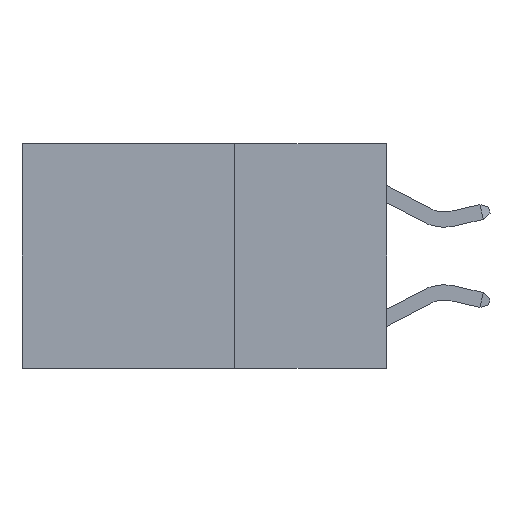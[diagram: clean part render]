
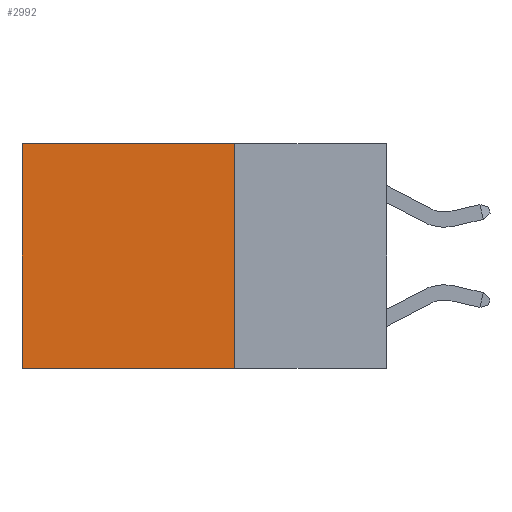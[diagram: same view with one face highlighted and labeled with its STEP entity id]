
A CAD part, left-side view. The second image highlights one B-rep face of the part: STEP entity #2992.
In plain terms, the highlighted planar face has unit normal (-1, 0, 0).
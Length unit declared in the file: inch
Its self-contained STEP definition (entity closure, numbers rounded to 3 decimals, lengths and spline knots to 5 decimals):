
#8 = VECTOR ( 'NONE', #3500, 39.37008 ) ;
#71 = VERTEX_POINT ( 'NONE', #1092 ) ;
#175 = ORIENTED_EDGE ( 'NONE', *, *, #10631, .F. ) ;
#311 = VECTOR ( 'NONE', #3768, 39.37008 ) ;
#1005 = LINE ( 'NONE', #7668, #5532 ) ;
#1092 = CARTESIAN_POINT ( 'NONE',  ( 0.2625, 0.25, -0.37 ) ) ;
#2127 = CARTESIAN_POINT ( 'NONE',  ( 0.2625, 0.25, 0. ) ) ;
#2194 = VERTEX_POINT ( 'NONE', #2640 ) ;
#2596 = CARTESIAN_POINT ( 'NONE',  ( 0.2625, 0.25, 0. ) ) ;
#2640 = CARTESIAN_POINT ( 'NONE',  ( 0.2625, 0.6, 0. ) ) ;
#2892 = ORIENTED_EDGE ( 'NONE', *, *, #11614, .T. ) ;
#2992 = ADVANCED_FACE ( 'NONE', ( #4055 ), #8138, .F. ) ;
#3033 = LINE ( 'NONE', #8359, #311 ) ;
#3107 = DIRECTION ( 'NONE',  ( 0., 1., 0. ) ) ;
#3500 = DIRECTION ( 'NONE',  ( 0., 0., -1. ) ) ;
#3768 = DIRECTION ( 'NONE',  ( 0., 1., 0. ) ) ;
#4055 = FACE_OUTER_BOUND ( 'NONE', #11778, .T. ) ;
#4772 = EDGE_CURVE ( 'NONE', #2194, #5757, #10464, .T. ) ;
#5532 = VECTOR ( 'NONE', #3107, 39.37008 ) ;
#5728 = EDGE_CURVE ( 'NONE', #71, #5757, #3033, .T. ) ;
#5757 = VERTEX_POINT ( 'NONE', #9264 ) ;
#6222 = AXIS2_PLACEMENT_3D ( 'NONE', #2127, #8356, #8332 ) ;
#6916 = ORIENTED_EDGE ( 'NONE', *, *, #4772, .T. ) ;
#7668 = CARTESIAN_POINT ( 'NONE',  ( 0.2625, 0.25, 0. ) ) ;
#8138 = PLANE ( 'NONE',  #6222 ) ;
#8252 = CARTESIAN_POINT ( 'NONE',  ( 0.2625, 0.25, 0. ) ) ;
#8332 = DIRECTION ( 'NONE',  ( 0., 0., -1. ) ) ;
#8356 = DIRECTION ( 'NONE',  ( 1., 0., 0. ) ) ;
#8359 = CARTESIAN_POINT ( 'NONE',  ( 0.2625, 0.25, -0.37 ) ) ;
#9264 = CARTESIAN_POINT ( 'NONE',  ( 0.2625, 0.6, -0.37 ) ) ;
#9647 = CARTESIAN_POINT ( 'NONE',  ( 0.2625, 0.6, 0. ) ) ;
#9749 = LINE ( 'NONE', #2596, #8 ) ;
#10182 = VECTOR ( 'NONE', #10555, 39.37008 ) ;
#10464 = LINE ( 'NONE', #9647, #10182 ) ;
#10555 = DIRECTION ( 'NONE',  ( 0., 0., -1. ) ) ;
#10631 = EDGE_CURVE ( 'NONE', #10769, #71, #9749, .T. ) ;
#10769 = VERTEX_POINT ( 'NONE', #8252 ) ;
#11614 = EDGE_CURVE ( 'NONE', #10769, #2194, #1005, .T. ) ;
#11720 = ORIENTED_EDGE ( 'NONE', *, *, #5728, .F. ) ;
#11778 = EDGE_LOOP ( 'NONE', ( #6916, #11720, #175, #2892 ) ) ;
